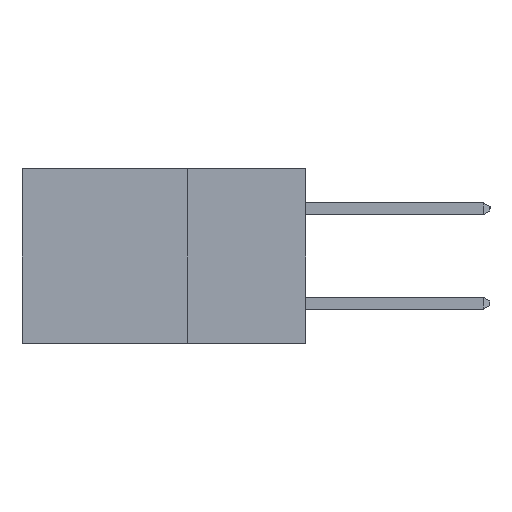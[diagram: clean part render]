
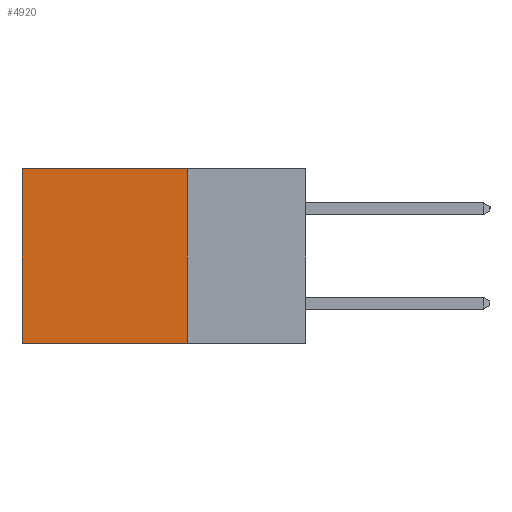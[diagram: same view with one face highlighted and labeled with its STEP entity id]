
A CAD part, left-side view. The second image highlights one B-rep face of the part: STEP entity #4920.
In plain terms, the highlighted planar face has unit normal (-1, 0, 0).
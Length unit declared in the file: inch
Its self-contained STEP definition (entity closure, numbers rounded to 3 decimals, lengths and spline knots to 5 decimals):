
#418 = CARTESIAN_POINT ( 'NONE',  ( 0.2615, 0.25, -0.37 ) ) ;
#610 = ORIENTED_EDGE ( 'NONE', *, *, #14306, .T. ) ;
#647 = ORIENTED_EDGE ( 'NONE', *, *, #18968, .F. ) ;
#713 = LINE ( 'NONE', #10307, #4190 ) ;
#1123 = CARTESIAN_POINT ( 'NONE',  ( 0.2615, 0.6, -0.37 ) ) ;
#2178 = VERTEX_POINT ( 'NONE', #17020 ) ;
#2199 = VECTOR ( 'NONE', #16540, 39.37008 ) ;
#2276 = LINE ( 'NONE', #3583, #5416 ) ;
#2305 = DIRECTION ( 'NONE',  ( 0., 1., 0. ) ) ;
#3399 = PLANE ( 'NONE',  #4164 ) ;
#3583 = CARTESIAN_POINT ( 'NONE',  ( 0.2615, 0.25, -0.37 ) ) ;
#3822 = EDGE_CURVE ( 'NONE', #8815, #2178, #713, .T. ) ;
#4164 = AXIS2_PLACEMENT_3D ( 'NONE', #418, #4830, #11006 ) ;
#4190 = VECTOR ( 'NONE', #2305, 39.37008 ) ;
#4435 = CARTESIAN_POINT ( 'NONE',  ( 0.2615, 0.25, -0.37 ) ) ;
#4619 = LINE ( 'NONE', #4435, #17631 ) ;
#4830 = DIRECTION ( 'NONE',  ( 1., 0., 0. ) ) ;
#4920 = ADVANCED_FACE ( 'NONE', ( #11096 ), #3399, .F. ) ;
#5416 = VECTOR ( 'NONE', #5500, 39.37008 ) ;
#5500 = DIRECTION ( 'NONE',  ( 0., 1., 0. ) ) ;
#5576 = EDGE_CURVE ( 'NONE', #14483, #17547, #2276, .T. ) ;
#5824 = CARTESIAN_POINT ( 'NONE',  ( 0.2615, 0.6, -0.37 ) ) ;
#7488 = LINE ( 'NONE', #1123, #2199 ) ;
#8815 = VERTEX_POINT ( 'NONE', #12108 ) ;
#10307 = CARTESIAN_POINT ( 'NONE',  ( 0.2615, 0.25, 0. ) ) ;
#11006 = DIRECTION ( 'NONE',  ( 0., 0., -1. ) ) ;
#11096 = FACE_OUTER_BOUND ( 'NONE', #16426, .T. ) ;
#12108 = CARTESIAN_POINT ( 'NONE',  ( 0.2615, 0.25, 0. ) ) ;
#12541 = CARTESIAN_POINT ( 'NONE',  ( 0.2615, 0.25, -0.37 ) ) ;
#14306 = EDGE_CURVE ( 'NONE', #2178, #17547, #7488, .T. ) ;
#14483 = VERTEX_POINT ( 'NONE', #12541 ) ;
#15021 = DIRECTION ( 'NONE',  ( 0., 0., -1. ) ) ;
#16426 = EDGE_LOOP ( 'NONE', ( #610, #19143, #647, #18590 ) ) ;
#16540 = DIRECTION ( 'NONE',  ( 0., 0., -1. ) ) ;
#17020 = CARTESIAN_POINT ( 'NONE',  ( 0.2615, 0.6, 0. ) ) ;
#17547 = VERTEX_POINT ( 'NONE', #5824 ) ;
#17631 = VECTOR ( 'NONE', #15021, 39.37008 ) ;
#18590 = ORIENTED_EDGE ( 'NONE', *, *, #3822, .T. ) ;
#18968 = EDGE_CURVE ( 'NONE', #8815, #14483, #4619, .T. ) ;
#19143 = ORIENTED_EDGE ( 'NONE', *, *, #5576, .F. ) ;
